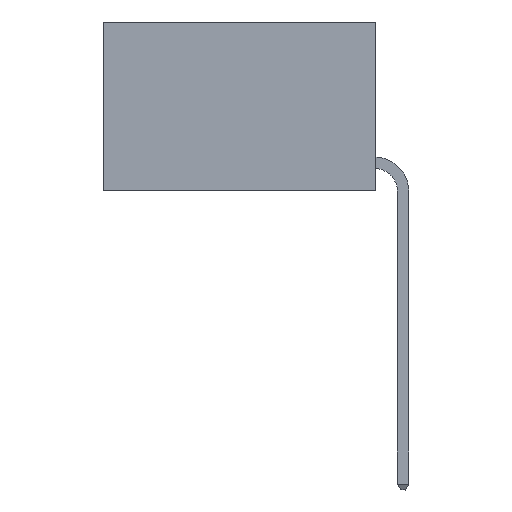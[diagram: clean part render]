
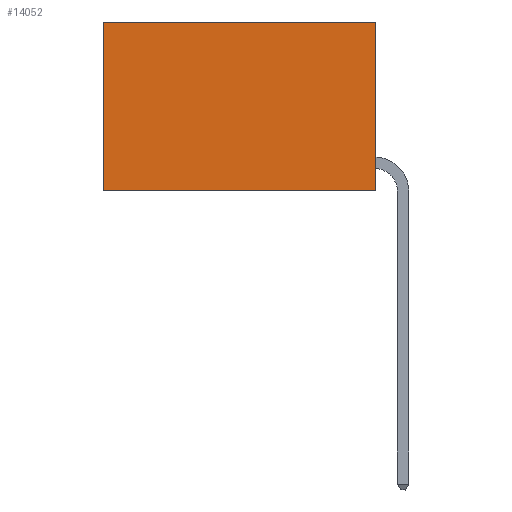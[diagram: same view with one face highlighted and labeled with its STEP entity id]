
A CAD part, left-side view. The second image highlights one B-rep face of the part: STEP entity #14052.
In plain terms, the highlighted planar face has unit normal (-1, 0, 0).
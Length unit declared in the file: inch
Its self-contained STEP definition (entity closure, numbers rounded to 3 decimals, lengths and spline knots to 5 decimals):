
#393 = ORIENTED_EDGE ( 'NONE', *, *, #5680, .T. ) ;
#987 = EDGE_CURVE ( 'NONE', #6062, #13535, #3589, .T. ) ;
#1891 = CARTESIAN_POINT ( 'NONE',  ( 0.2625, 0.6, 0. ) ) ;
#1894 = EDGE_CURVE ( 'NONE', #10108, #12819, #6726, .T. ) ;
#2968 = ORIENTED_EDGE ( 'NONE', *, *, #987, .T. ) ;
#3033 = VECTOR ( 'NONE', #7490, 39.37008 ) ;
#3303 = DIRECTION ( 'NONE',  ( 0., 0., -1. ) ) ;
#3589 = LINE ( 'NONE', #16081, #7549 ) ;
#3946 = DIRECTION ( 'NONE',  ( 0., 0., -1. ) ) ;
#4029 = LINE ( 'NONE', #1891, #17131 ) ;
#4201 = FACE_OUTER_BOUND ( 'NONE', #9876, .T. ) ;
#4460 = CARTESIAN_POINT ( 'NONE',  ( 0.2625, 0., -0.37 ) ) ;
#4474 = ORIENTED_EDGE ( 'NONE', *, *, #10832, .F. ) ;
#4852 = CARTESIAN_POINT ( 'NONE',  ( 0.2625, 0.6, 0. ) ) ;
#5680 = EDGE_CURVE ( 'NONE', #13535, #12819, #4029, .T. ) ;
#6062 = VERTEX_POINT ( 'NONE', #11863 ) ;
#6110 = CARTESIAN_POINT ( 'NONE',  ( 0.2625, 0.6, -0.37 ) ) ;
#6315 = VECTOR ( 'NONE', #12715, 39.37008 ) ;
#6726 = LINE ( 'NONE', #9098, #6315 ) ;
#7490 = DIRECTION ( 'NONE',  ( 0., 0., -1. ) ) ;
#7549 = VECTOR ( 'NONE', #8577, 39.37008 ) ;
#8577 = DIRECTION ( 'NONE',  ( 0., 1., 0. ) ) ;
#8751 = AXIS2_PLACEMENT_3D ( 'NONE', #16999, #11794, #3946 ) ;
#9098 = CARTESIAN_POINT ( 'NONE',  ( 0.2625, 0., -0.37 ) ) ;
#9876 = EDGE_LOOP ( 'NONE', ( #393, #14507, #4474, #2968 ) ) ;
#10104 = CARTESIAN_POINT ( 'NONE',  ( 0.2625, 0., 0. ) ) ;
#10108 = VERTEX_POINT ( 'NONE', #4460 ) ;
#10832 = EDGE_CURVE ( 'NONE', #6062, #10108, #16614, .T. ) ;
#11734 = PLANE ( 'NONE',  #8751 ) ;
#11794 = DIRECTION ( 'NONE',  ( 1., 0., 0. ) ) ;
#11863 = CARTESIAN_POINT ( 'NONE',  ( 0.2625, 0., 0. ) ) ;
#12715 = DIRECTION ( 'NONE',  ( 0., 1., 0. ) ) ;
#12819 = VERTEX_POINT ( 'NONE', #6110 ) ;
#13535 = VERTEX_POINT ( 'NONE', #4852 ) ;
#14052 = ADVANCED_FACE ( 'NONE', ( #4201 ), #11734, .F. ) ;
#14507 = ORIENTED_EDGE ( 'NONE', *, *, #1894, .F. ) ;
#16081 = CARTESIAN_POINT ( 'NONE',  ( 0.2625, 0., 0. ) ) ;
#16614 = LINE ( 'NONE', #10104, #3033 ) ;
#16999 = CARTESIAN_POINT ( 'NONE',  ( 0.2625, 0., 0. ) ) ;
#17131 = VECTOR ( 'NONE', #3303, 39.37008 ) ;
